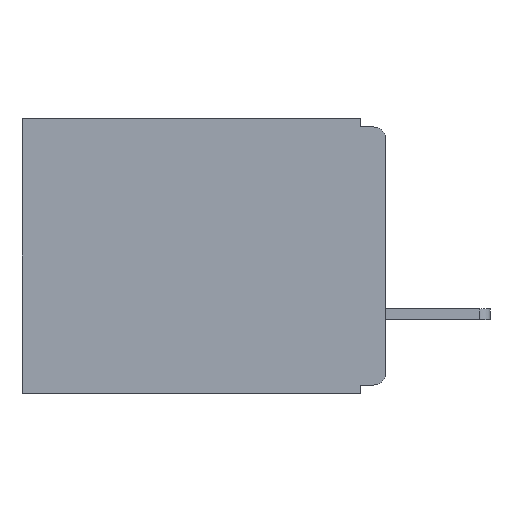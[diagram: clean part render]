
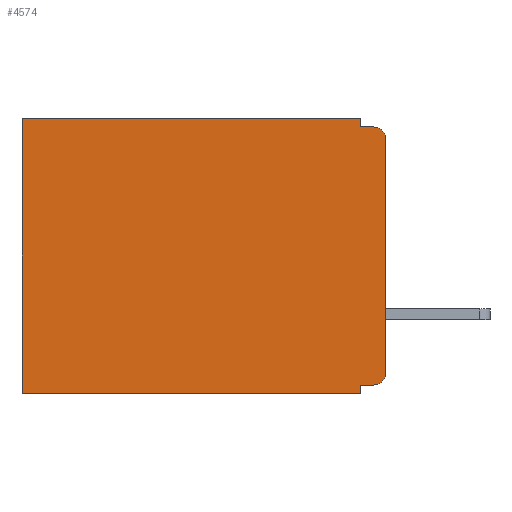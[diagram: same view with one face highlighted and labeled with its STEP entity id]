
A CAD part, left-side view. The second image highlights one B-rep face of the part: STEP entity #4574.
In plain terms, the highlighted planar face has unit normal (-1, 0, 0).
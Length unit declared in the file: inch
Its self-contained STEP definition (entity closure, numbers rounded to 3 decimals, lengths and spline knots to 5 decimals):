
#722 = VERTEX_POINT ( 'NONE', #11270 ) ;
#1192 = VECTOR ( 'NONE', #6497, 39.37008 ) ;
#1263 = EDGE_CURVE ( 'NONE', #8497, #4280, #4063, .T. ) ;
#1393 = CARTESIAN_POINT ( 'NONE',  ( 0.3, 0., -0.33 ) ) ;
#1990 = LINE ( 'NONE', #8278, #11859 ) ;
#2113 = EDGE_LOOP ( 'NONE', ( #10040, #3720, #5026, #5313, #6789, #7912, #8135, #8157, #8971, #9839 ) ) ;
#2876 = VECTOR ( 'NONE', #12286, 39.37008 ) ;
#2902 = CIRCLE ( 'NONE', #3778, 0.015 ) ;
#2997 = VERTEX_POINT ( 'NONE', #11613 ) ;
#3016 = VECTOR ( 'NONE', #12454, 39.37008 ) ;
#3034 = DIRECTION ( 'NONE',  ( 0., 0., -1. ) ) ;
#3601 = DIRECTION ( 'NONE',  ( 0., 1., 0. ) ) ;
#3720 = ORIENTED_EDGE ( 'NONE', *, *, #9041, .T. ) ;
#3778 = AXIS2_PLACEMENT_3D ( 'NONE', #5679, #11934, #6684 ) ;
#3802 = VECTOR ( 'NONE', #3601, 39.37008 ) ;
#4062 = AXIS2_PLACEMENT_3D ( 'NONE', #10299, #4544, #11117 ) ;
#4063 = LINE ( 'NONE', #11639, #3802 ) ;
#4279 = VERTEX_POINT ( 'NONE', #6201 ) ;
#4280 = VERTEX_POINT ( 'NONE', #6279 ) ;
#4313 = CARTESIAN_POINT ( 'NONE',  ( 0.3, 0.031, -0.33 ) ) ;
#4475 = DIRECTION ( 'NONE',  ( 1., 0., 0. ) ) ;
#4543 = DIRECTION ( 'NONE',  ( 0., 0., -1. ) ) ;
#4544 = DIRECTION ( 'NONE',  ( -1., 0., 0. ) ) ;
#4574 = ADVANCED_FACE ( 'NONE', ( #5144 ), #7689, .F. ) ;
#4610 = VERTEX_POINT ( 'NONE', #8911 ) ;
#4734 = EDGE_CURVE ( 'NONE', #4280, #4279, #5641, .T. ) ;
#5026 = ORIENTED_EDGE ( 'NONE', *, *, #8892, .F. ) ;
#5143 = VECTOR ( 'NONE', #9255, 39.37008 ) ;
#5144 = FACE_OUTER_BOUND ( 'NONE', #2113, .T. ) ;
#5313 = ORIENTED_EDGE ( 'NONE', *, *, #10118, .F. ) ;
#5468 = LINE ( 'NONE', #4313, #5143 ) ;
#5546 = CARTESIAN_POINT ( 'NONE',  ( 0.3, 0.015, -0.01 ) ) ;
#5641 = LINE ( 'NONE', #12384, #10367 ) ;
#5663 = LINE ( 'NONE', #11520, #2876 ) ;
#5679 = CARTESIAN_POINT ( 'NONE',  ( 0.3, 0.015, -0.305 ) ) ;
#5689 = CARTESIAN_POINT ( 'NONE',  ( 0.3, 0.031, 0. ) ) ;
#6201 = CARTESIAN_POINT ( 'NONE',  ( 0.3, 0.437, -0.33 ) ) ;
#6279 = CARTESIAN_POINT ( 'NONE',  ( 0.3, 0.437, 0. ) ) ;
#6379 = CARTESIAN_POINT ( 'NONE',  ( 0.3, 0.031, 0. ) ) ;
#6497 = DIRECTION ( 'NONE',  ( 0., 1., 0. ) ) ;
#6684 = DIRECTION ( 'NONE',  ( 0., 0., -1. ) ) ;
#6789 = ORIENTED_EDGE ( 'NONE', *, *, #1263, .T. ) ;
#7420 = VERTEX_POINT ( 'NONE', #10274 ) ;
#7689 = PLANE ( 'NONE',  #11865 ) ;
#7770 = DIRECTION ( 'NONE',  ( 0., 0., -1. ) ) ;
#7912 = ORIENTED_EDGE ( 'NONE', *, *, #4734, .T. ) ;
#8135 = ORIENTED_EDGE ( 'NONE', *, *, #9974, .F. ) ;
#8157 = ORIENTED_EDGE ( 'NONE', *, *, #10132, .F. ) ;
#8278 = CARTESIAN_POINT ( 'NONE',  ( 0.3, 0., -0.01 ) ) ;
#8307 = CIRCLE ( 'NONE', #4062, 0.015 ) ;
#8497 = VERTEX_POINT ( 'NONE', #5689 ) ;
#8751 = VECTOR ( 'NONE', #3034, 39.37008 ) ;
#8768 = EDGE_CURVE ( 'NONE', #11683, #4610, #11030, .T. ) ;
#8892 = EDGE_CURVE ( 'NONE', #7420, #9020, #1990, .T. ) ;
#8911 = CARTESIAN_POINT ( 'NONE',  ( 0.3, 0., -0.305 ) ) ;
#8971 = ORIENTED_EDGE ( 'NONE', *, *, #8993, .F. ) ;
#8993 = EDGE_CURVE ( 'NONE', #9570, #2997, #10907, .T. ) ;
#9020 = VERTEX_POINT ( 'NONE', #5546 ) ;
#9041 = EDGE_CURVE ( 'NONE', #11683, #9020, #8307, .T. ) ;
#9107 = EDGE_CURVE ( 'NONE', #9570, #4610, #2902, .T. ) ;
#9255 = DIRECTION ( 'NONE',  ( 0., 0., -1. ) ) ;
#9373 = CARTESIAN_POINT ( 'NONE',  ( 0.3, 0.015, -0.32 ) ) ;
#9570 = VERTEX_POINT ( 'NONE', #9373 ) ;
#9839 = ORIENTED_EDGE ( 'NONE', *, *, #9107, .T. ) ;
#9974 = EDGE_CURVE ( 'NONE', #722, #4279, #5663, .T. ) ;
#10040 = ORIENTED_EDGE ( 'NONE', *, *, #8768, .F. ) ;
#10118 = EDGE_CURVE ( 'NONE', #8497, #7420, #12502, .T. ) ;
#10132 = EDGE_CURVE ( 'NONE', #2997, #722, #5468, .T. ) ;
#10274 = CARTESIAN_POINT ( 'NONE',  ( 0.3, 0.031, -0.01 ) ) ;
#10299 = CARTESIAN_POINT ( 'NONE',  ( 0.3, 0.015, -0.025 ) ) ;
#10367 = VECTOR ( 'NONE', #7770, 39.37008 ) ;
#10703 = CARTESIAN_POINT ( 'NONE',  ( 0.3, 0., -0.33 ) ) ;
#10907 = LINE ( 'NONE', #11801, #1192 ) ;
#10908 = DIRECTION ( 'NONE',  ( 0., -1., 0. ) ) ;
#11030 = LINE ( 'NONE', #10703, #8751 ) ;
#11117 = DIRECTION ( 'NONE',  ( 0., 0., -1. ) ) ;
#11189 = CARTESIAN_POINT ( 'NONE',  ( 0.3, 0., -0.025 ) ) ;
#11270 = CARTESIAN_POINT ( 'NONE',  ( 0.3, 0.031, -0.33 ) ) ;
#11520 = CARTESIAN_POINT ( 'NONE',  ( 0.3, 0., -0.33 ) ) ;
#11613 = CARTESIAN_POINT ( 'NONE',  ( 0.3, 0.031, -0.32 ) ) ;
#11639 = CARTESIAN_POINT ( 'NONE',  ( 0.3, 0., 0. ) ) ;
#11683 = VERTEX_POINT ( 'NONE', #11189 ) ;
#11801 = CARTESIAN_POINT ( 'NONE',  ( 0.3, 0., -0.32 ) ) ;
#11859 = VECTOR ( 'NONE', #10908, 39.37008 ) ;
#11865 = AXIS2_PLACEMENT_3D ( 'NONE', #1393, #4475, #4543 ) ;
#11934 = DIRECTION ( 'NONE',  ( -1., 0., 0. ) ) ;
#12286 = DIRECTION ( 'NONE',  ( 0., 1., 0. ) ) ;
#12384 = CARTESIAN_POINT ( 'NONE',  ( 0.3, 0.437, -0.33 ) ) ;
#12454 = DIRECTION ( 'NONE',  ( 0., 0., -1. ) ) ;
#12502 = LINE ( 'NONE', #6379, #3016 ) ;
